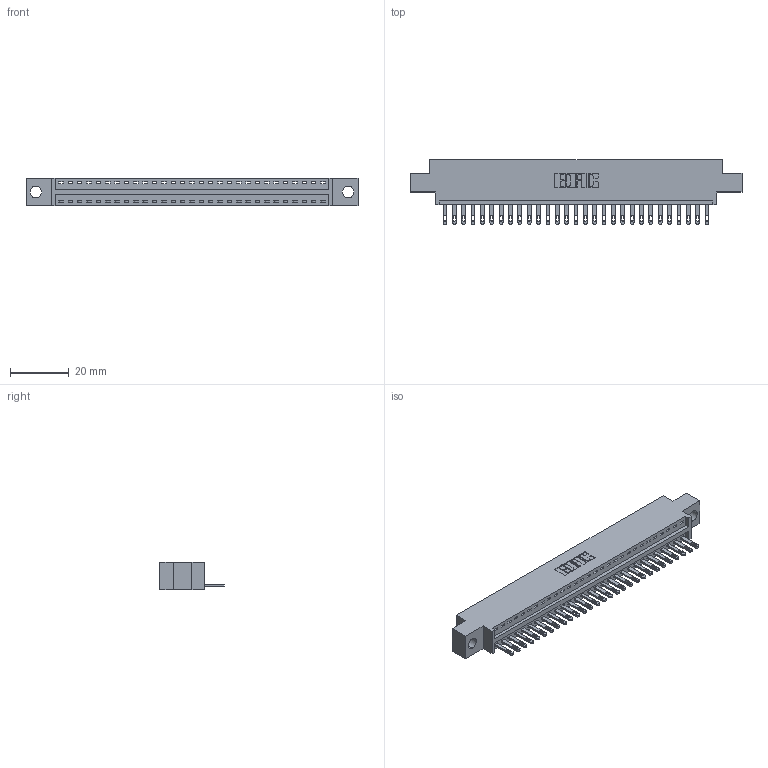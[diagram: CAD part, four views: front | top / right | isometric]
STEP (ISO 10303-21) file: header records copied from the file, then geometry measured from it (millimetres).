
FILE_DESCRIPTION (( 'STEP AP203' ), '1' );
FILE_NAME ('346-029-500-604.STEP', '2018-08-22T02:57:13', ( '' ), ( '' ), 'SwSTEP 2.0', 'SolidWorks 2016', '' );
FILE_SCHEMA (( 'CONFIG_CONTROL_DESIGN' ));
Length unit declared in the file: inch
Products named in the file (3): 346-029-500-604; 346 Part_0.170 Offset - 0.156 Dia-TH; 345-292-001_345-293-100
Assembly tree (30 placements, depth 2):
  346-029-500-604
    346 Part_0.170 Offset - 0.156 Dia-TH
    345-292-001_345-293-100  x29
Bounding box: 112.65 x 21.84 x 9.4 mm (x, y, z)
Volume: 10468.9 mm3; surface area: 12977.4 mm2
Topology: 30 solids, 30 shells, 1692 faces, 5213 edges, 3474 vertices
Faces by surface type: plane 1066, cylinder 626
Entity records: 19813 total; most frequent: CARTESIAN_POINT 3407, ORIENTED_EDGE 3370, DIRECTION 3023, EDGE_CURVE 1685, LINE 1433, VECTOR 1433, VERTEX_POINT 1122, AXIS2_PLACEMENT_3D 795
